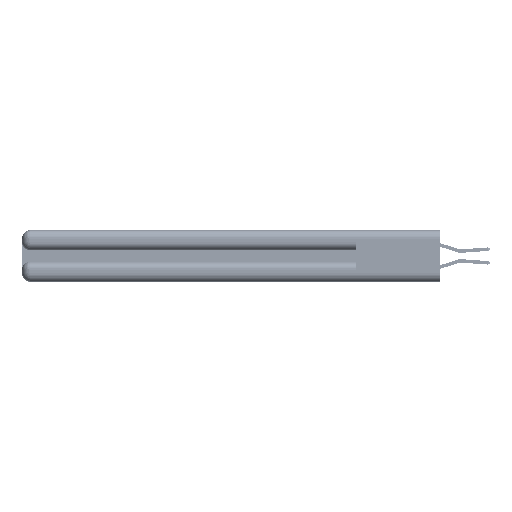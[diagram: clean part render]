
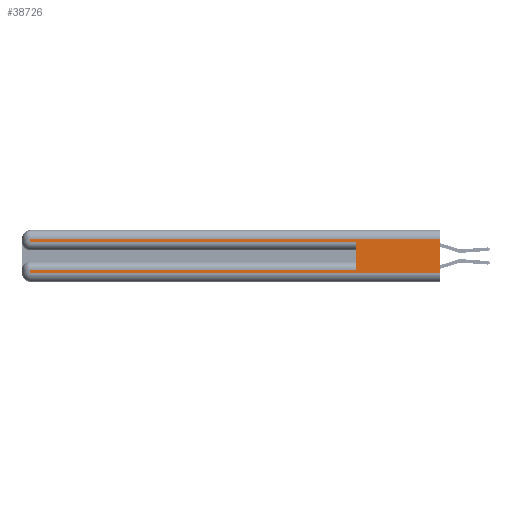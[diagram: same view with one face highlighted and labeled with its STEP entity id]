
A CAD part, left-side view. The second image highlights one B-rep face of the part: STEP entity #38726.
In plain terms, the highlighted planar face has unit normal (-1, 0, 0).
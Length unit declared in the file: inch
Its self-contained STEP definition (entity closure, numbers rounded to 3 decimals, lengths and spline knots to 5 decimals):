
#307 = DIRECTION ( 'NONE',  ( 0., 0., 1. ) ) ;
#726 = EDGE_CURVE ( 'NONE', #45923, #17257, #12578, .T. ) ;
#1160 = CARTESIAN_POINT ( 'NONE',  ( 0., 0., 0.285 ) ) ;
#1374 = CARTESIAN_POINT ( 'NONE',  ( 0., 0., 0.085 ) ) ;
#1389 = CARTESIAN_POINT ( 'NONE',  ( 0., 2.94, 0.37 ) ) ;
#3542 = PLANE ( 'NONE',  #26017 ) ;
#4108 = LINE ( 'NONE', #1374, #18360 ) ;
#4728 = CARTESIAN_POINT ( 'NONE',  ( 0., 0.6, 0.085 ) ) ;
#4951 = EDGE_CURVE ( 'NONE', #28602, #9457, #13100, .T. ) ;
#6496 = EDGE_CURVE ( 'NONE', #48603, #19632, #9784, .T. ) ;
#8120 = ORIENTED_EDGE ( 'NONE', *, *, #4951, .T. ) ;
#8702 = EDGE_CURVE ( 'NONE', #45923, #48603, #4108, .T. ) ;
#9457 = VERTEX_POINT ( 'NONE', #10422 ) ;
#9784 = LINE ( 'NONE', #1389, #17295 ) ;
#10422 = CARTESIAN_POINT ( 'NONE',  ( 0., 2.94, 0.31 ) ) ;
#10697 = CARTESIAN_POINT ( 'NONE',  ( 0., 0., 0.06 ) ) ;
#11300 = VERTEX_POINT ( 'NONE', #10697 ) ;
#12578 = LINE ( 'NONE', #12920, #28879 ) ;
#12920 = CARTESIAN_POINT ( 'NONE',  ( 0., 0.6, 0.145 ) ) ;
#13100 = LINE ( 'NONE', #24809, #16861 ) ;
#14316 = DIRECTION ( 'NONE',  ( 0., -1., 0. ) ) ;
#14601 = EDGE_CURVE ( 'NONE', #9457, #20697, #45961, .T. ) ;
#14949 = LINE ( 'NONE', #26426, #25025 ) ;
#15635 = DIRECTION ( 'NONE',  ( 1., 0., 0. ) ) ;
#16572 = ORIENTED_EDGE ( 'NONE', *, *, #8702, .T. ) ;
#16861 = VECTOR ( 'NONE', #37054, 39.37008 ) ;
#17257 = VERTEX_POINT ( 'NONE', #23088 ) ;
#17262 = CARTESIAN_POINT ( 'NONE',  ( 0., 2.94, 0.06 ) ) ;
#17295 = VECTOR ( 'NONE', #29454, 39.37008 ) ;
#17471 = CARTESIAN_POINT ( 'NONE',  ( 0., 2.94, 0.37 ) ) ;
#17529 = CARTESIAN_POINT ( 'NONE',  ( 0., 0., 0.31 ) ) ;
#18328 = ORIENTED_EDGE ( 'NONE', *, *, #14601, .T. ) ;
#18360 = VECTOR ( 'NONE', #33460, 39.37008 ) ;
#18629 = VECTOR ( 'NONE', #20844, 39.37008 ) ;
#18996 = EDGE_CURVE ( 'NONE', #19632, #11300, #14949, .T. ) ;
#19632 = VERTEX_POINT ( 'NONE', #17262 ) ;
#19982 = CARTESIAN_POINT ( 'NONE',  ( 0., 0., 0.37 ) ) ;
#20697 = VERTEX_POINT ( 'NONE', #50861 ) ;
#20844 = DIRECTION ( 'NONE',  ( 0., 0., -1. ) ) ;
#23088 = CARTESIAN_POINT ( 'NONE',  ( 0., 0.6, 0.285 ) ) ;
#24721 = ORIENTED_EDGE ( 'NONE', *, *, #6496, .T. ) ;
#24809 = CARTESIAN_POINT ( 'NONE',  ( 0., 0., 0.31 ) ) ;
#25025 = VECTOR ( 'NONE', #14316, 39.37008 ) ;
#26017 = AXIS2_PLACEMENT_3D ( 'NONE', #19982, #15635, #39630 ) ;
#26426 = CARTESIAN_POINT ( 'NONE',  ( 0., 0., 0.06 ) ) ;
#26714 = EDGE_CURVE ( 'NONE', #28602, #11300, #31343, .T. ) ;
#27165 = VECTOR ( 'NONE', #33404, 39.37008 ) ;
#28602 = VERTEX_POINT ( 'NONE', #17529 ) ;
#28879 = VECTOR ( 'NONE', #307, 39.37008 ) ;
#29454 = DIRECTION ( 'NONE',  ( 0., 0., -1. ) ) ;
#30064 = DIRECTION ( 'NONE',  ( 0., 0., -1. ) ) ;
#31343 = LINE ( 'NONE', #44819, #18629 ) ;
#33404 = DIRECTION ( 'NONE',  ( 0., -1., 0. ) ) ;
#33460 = DIRECTION ( 'NONE',  ( 0., 1., 0. ) ) ;
#33535 = FACE_OUTER_BOUND ( 'NONE', #34896, .T. ) ;
#34896 = EDGE_LOOP ( 'NONE', ( #42062, #8120, #18328, #35961, #48399, #16572, #24721, #39314 ) ) ;
#35961 = ORIENTED_EDGE ( 'NONE', *, *, #46737, .T. ) ;
#37054 = DIRECTION ( 'NONE',  ( 0., 1., 0. ) ) ;
#38726 = ADVANCED_FACE ( 'NONE', ( #33535 ), #3542, .F. ) ;
#39314 = ORIENTED_EDGE ( 'NONE', *, *, #18996, .T. ) ;
#39630 = DIRECTION ( 'NONE',  ( 0., 0., -1. ) ) ;
#40930 = VECTOR ( 'NONE', #30064, 39.37008 ) ;
#42062 = ORIENTED_EDGE ( 'NONE', *, *, #26714, .F. ) ;
#44819 = CARTESIAN_POINT ( 'NONE',  ( 0., 0., 0.37 ) ) ;
#45923 = VERTEX_POINT ( 'NONE', #4728 ) ;
#45961 = LINE ( 'NONE', #17471, #40930 ) ;
#46737 = EDGE_CURVE ( 'NONE', #20697, #17257, #47851, .T. ) ;
#47851 = LINE ( 'NONE', #1160, #27165 ) ;
#48205 = CARTESIAN_POINT ( 'NONE',  ( 0., 2.94, 0.085 ) ) ;
#48399 = ORIENTED_EDGE ( 'NONE', *, *, #726, .F. ) ;
#48603 = VERTEX_POINT ( 'NONE', #48205 ) ;
#50861 = CARTESIAN_POINT ( 'NONE',  ( 0., 2.94, 0.285 ) ) ;
